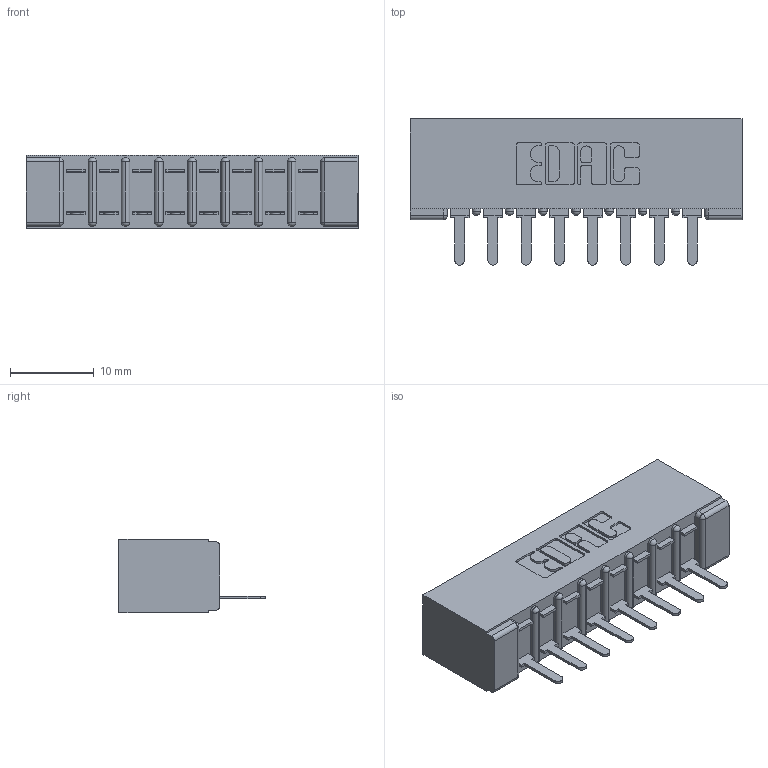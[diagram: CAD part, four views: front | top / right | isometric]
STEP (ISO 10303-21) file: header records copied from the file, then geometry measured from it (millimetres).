
FILE_DESCRIPTION (( 'STEP AP203' ), '1' );
FILE_NAME ('307-008-521-101.STEP', '2019-09-04T18:24:30', ( '' ), ( '' ), 'SwSTEP 2.0', 'SolidWorks 2016', '' );
FILE_SCHEMA (( 'CONFIG_CONTROL_DESIGN' ));
Length unit declared in the file: inch
Products named in the file (3): 307 Part_No Mounting Lugs; 307-008-521-101; 307-290-002_521
Assembly tree (9 placements, depth 2):
  307-008-521-101
    307 Part_No Mounting Lugs
    307-290-002_521  x8
Bounding box: 39.57 x 17.42 x 8.71 mm (x, y, z)
Volume: 2848 mm3; surface area: 4913.6 mm2
Topology: 9 solids, 9 shells, 711 faces, 2155 edges, 1410 vertices
Faces by surface type: plane 426, cylinder 267, sphere 18
Entity records: 11490 total; most frequent: CARTESIAN_POINT 1932, ORIENTED_EDGE 1922, DIRECTION 1891, EDGE_CURVE 961, VECTOR 721, LINE 721, VERTEX_POINT 626, AXIS2_PLACEMENT_3D 585
